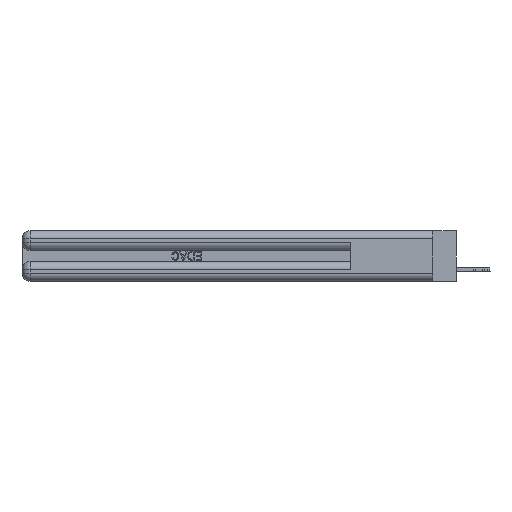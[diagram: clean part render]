
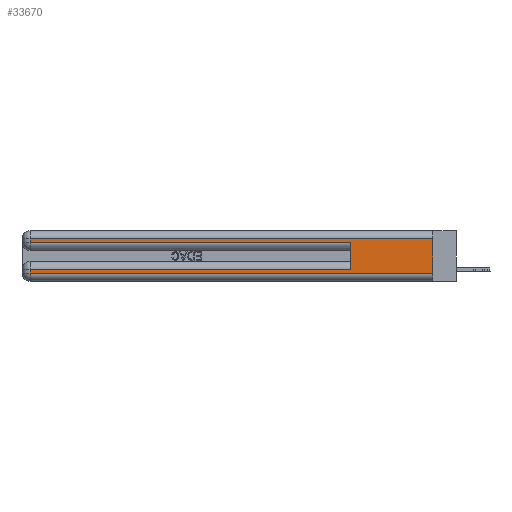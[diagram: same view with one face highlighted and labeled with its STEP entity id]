
A CAD part, left-side view. The second image highlights one B-rep face of the part: STEP entity #33670.
In plain terms, the highlighted planar face has unit normal (-1, 0, 0).
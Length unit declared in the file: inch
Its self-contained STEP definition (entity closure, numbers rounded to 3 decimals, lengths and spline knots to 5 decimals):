
#355 = ORIENTED_EDGE ( 'NONE', *, *, #20141, .T. ) ;
#1056 = CARTESIAN_POINT ( 'NONE',  ( 0., 2.94, 0.31 ) ) ;
#1088 = DIRECTION ( 'NONE',  ( 0., 0., -1. ) ) ;
#2325 = CARTESIAN_POINT ( 'NONE',  ( 0., 2.94, 0.285 ) ) ;
#2327 = DIRECTION ( 'NONE',  ( 0., -1., 0. ) ) ;
#3626 = EDGE_CURVE ( 'NONE', #27557, #28989, #27286, .T. ) ;
#6007 = DIRECTION ( 'NONE',  ( 0., 1., 0. ) ) ;
#8840 = ORIENTED_EDGE ( 'NONE', *, *, #3626, .T. ) ;
#9269 = EDGE_CURVE ( 'NONE', #20031, #28989, #42678, .T. ) ;
#9508 = VECTOR ( 'NONE', #45151, 39.37008 ) ;
#9889 = VERTEX_POINT ( 'NONE', #41621 ) ;
#10449 = CARTESIAN_POINT ( 'NONE',  ( 0., 2.94, 0.37 ) ) ;
#10870 = LINE ( 'NONE', #44864, #18041 ) ;
#12458 = VERTEX_POINT ( 'NONE', #48445 ) ;
#13232 = CARTESIAN_POINT ( 'NONE',  ( 0., 0., 0.285 ) ) ;
#14266 = ORIENTED_EDGE ( 'NONE', *, *, #24169, .T. ) ;
#14810 = CARTESIAN_POINT ( 'NONE',  ( 0., 2.94, 0.37 ) ) ;
#17286 = CARTESIAN_POINT ( 'NONE',  ( 0., 0., 0.31 ) ) ;
#17709 = CARTESIAN_POINT ( 'NONE',  ( 0., 0.6, 0.145 ) ) ;
#18041 = VECTOR ( 'NONE', #35053, 39.37008 ) ;
#19869 = LINE ( 'NONE', #14810, #30872 ) ;
#20031 = VERTEX_POINT ( 'NONE', #40345 ) ;
#20141 = EDGE_CURVE ( 'NONE', #24881, #35769, #42003, .T. ) ;
#20327 = FACE_OUTER_BOUND ( 'NONE', #28240, .T. ) ;
#21993 = AXIS2_PLACEMENT_3D ( 'NONE', #35480, #39171, #1088 ) ;
#22501 = DIRECTION ( 'NONE',  ( 0., 0., -1. ) ) ;
#23845 = VECTOR ( 'NONE', #6007, 39.37008 ) ;
#24169 = EDGE_CURVE ( 'NONE', #36857, #12458, #36711, .T. ) ;
#24519 = LINE ( 'NONE', #47633, #47396 ) ;
#24881 = VERTEX_POINT ( 'NONE', #17286 ) ;
#25089 = DIRECTION ( 'NONE',  ( 0., -1., 0. ) ) ;
#25904 = LINE ( 'NONE', #33678, #38607 ) ;
#27286 = LINE ( 'NONE', #13232, #33955 ) ;
#27557 = VERTEX_POINT ( 'NONE', #2325 ) ;
#28090 = ORIENTED_EDGE ( 'NONE', *, *, #37259, .T. ) ;
#28240 = EDGE_LOOP ( 'NONE', ( #32988, #355, #28090, #8840, #42628, #34014, #14266, #47474 ) ) ;
#28354 = DIRECTION ( 'NONE',  ( 0., 0., 1. ) ) ;
#28989 = VERTEX_POINT ( 'NONE', #49544 ) ;
#30872 = VECTOR ( 'NONE', #41150, 39.37008 ) ;
#31476 = EDGE_CURVE ( 'NONE', #20031, #36857, #10870, .T. ) ;
#32988 = ORIENTED_EDGE ( 'NONE', *, *, #46262, .F. ) ;
#33670 = ADVANCED_FACE ( 'NONE', ( #20327 ), #43200, .F. ) ;
#33678 = CARTESIAN_POINT ( 'NONE',  ( 0., 0., 0.37 ) ) ;
#33955 = VECTOR ( 'NONE', #2327, 39.37008 ) ;
#34014 = ORIENTED_EDGE ( 'NONE', *, *, #31476, .T. ) ;
#35053 = DIRECTION ( 'NONE',  ( 0., 1., 0. ) ) ;
#35480 = CARTESIAN_POINT ( 'NONE',  ( 0., 0., 0.37 ) ) ;
#35769 = VERTEX_POINT ( 'NONE', #1056 ) ;
#36711 = LINE ( 'NONE', #10449, #9508 ) ;
#36857 = VERTEX_POINT ( 'NONE', #46149 ) ;
#37259 = EDGE_CURVE ( 'NONE', #35769, #27557, #19869, .T. ) ;
#38535 = VECTOR ( 'NONE', #28354, 39.37008 ) ;
#38607 = VECTOR ( 'NONE', #22501, 39.37008 ) ;
#39171 = DIRECTION ( 'NONE',  ( 1., 0., 0. ) ) ;
#40345 = CARTESIAN_POINT ( 'NONE',  ( 0., 0.6, 0.085 ) ) ;
#41150 = DIRECTION ( 'NONE',  ( 0., 0., -1. ) ) ;
#41621 = CARTESIAN_POINT ( 'NONE',  ( 0., 0., 0.06 ) ) ;
#42003 = LINE ( 'NONE', #43743, #23845 ) ;
#42628 = ORIENTED_EDGE ( 'NONE', *, *, #9269, .F. ) ;
#42678 = LINE ( 'NONE', #17709, #38535 ) ;
#43200 = PLANE ( 'NONE',  #21993 ) ;
#43743 = CARTESIAN_POINT ( 'NONE',  ( 0., 0., 0.31 ) ) ;
#44864 = CARTESIAN_POINT ( 'NONE',  ( 0., 0., 0.085 ) ) ;
#45151 = DIRECTION ( 'NONE',  ( 0., 0., -1. ) ) ;
#46149 = CARTESIAN_POINT ( 'NONE',  ( 0., 2.94, 0.085 ) ) ;
#46262 = EDGE_CURVE ( 'NONE', #24881, #9889, #25904, .T. ) ;
#47377 = EDGE_CURVE ( 'NONE', #12458, #9889, #24519, .T. ) ;
#47396 = VECTOR ( 'NONE', #25089, 39.37008 ) ;
#47474 = ORIENTED_EDGE ( 'NONE', *, *, #47377, .T. ) ;
#47633 = CARTESIAN_POINT ( 'NONE',  ( 0., 0., 0.06 ) ) ;
#48445 = CARTESIAN_POINT ( 'NONE',  ( 0., 2.94, 0.06 ) ) ;
#49544 = CARTESIAN_POINT ( 'NONE',  ( 0., 0.6, 0.285 ) ) ;
